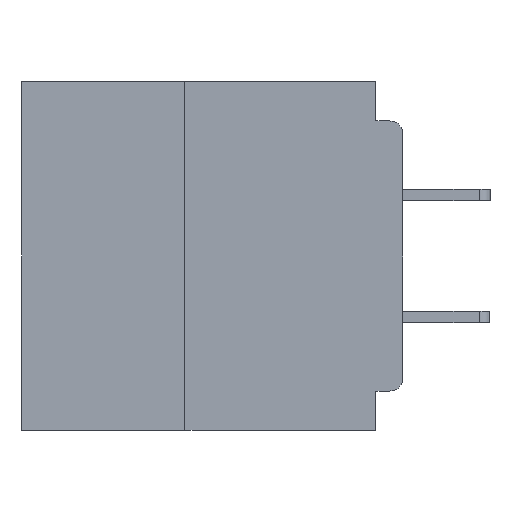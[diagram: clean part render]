
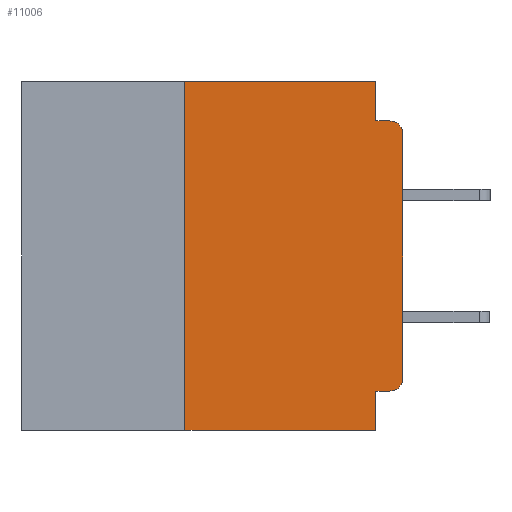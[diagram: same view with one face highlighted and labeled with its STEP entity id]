
A CAD part, left-side view. The second image highlights one B-rep face of the part: STEP entity #11006.
In plain terms, the highlighted planar face has unit normal (-1, 0, 0).
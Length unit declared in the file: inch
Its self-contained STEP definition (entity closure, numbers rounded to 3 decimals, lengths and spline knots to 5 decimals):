
#966 = CIRCLE ( 'NONE', #8583, 0.015 ) ;
#2147 = CARTESIAN_POINT ( 'NONE',  ( 0., 0.031, -0.045 ) ) ;
#2228 = ORIENTED_EDGE ( 'NONE', *, *, #18064, .T. ) ;
#3754 = CARTESIAN_POINT ( 'NONE',  ( 0., 0., -0.34 ) ) ;
#4077 = VERTEX_POINT ( 'NONE', #32138 ) ;
#4390 = LINE ( 'NONE', #18582, #49183 ) ;
#4826 = LINE ( 'NONE', #20694, #47069 ) ;
#5612 = CARTESIAN_POINT ( 'NONE',  ( 0., 0., -0.355 ) ) ;
#6241 = CARTESIAN_POINT ( 'NONE',  ( 0., 0.031, 0. ) ) ;
#7669 = ORIENTED_EDGE ( 'NONE', *, *, #29895, .F. ) ;
#7834 = LINE ( 'NONE', #51742, #28406 ) ;
#7839 = VERTEX_POINT ( 'NONE', #52609 ) ;
#7979 = LINE ( 'NONE', #29197, #25953 ) ;
#8038 = VECTOR ( 'NONE', #11817, 39.37008 ) ;
#8240 = EDGE_CURVE ( 'NONE', #22325, #8984, #49667, .T. ) ;
#8583 = AXIS2_PLACEMENT_3D ( 'NONE', #45046, #20536, #49139 ) ;
#8984 = VERTEX_POINT ( 'NONE', #2147 ) ;
#10341 = DIRECTION ( 'NONE',  ( 0., 0., -1. ) ) ;
#11006 = ADVANCED_FACE ( 'NONE', ( #14871 ), #15702, .F. ) ;
#11491 = AXIS2_PLACEMENT_3D ( 'NONE', #27928, #44354, #19817 ) ;
#11817 = DIRECTION ( 'NONE',  ( 0., -1., 0. ) ) ;
#12383 = LINE ( 'NONE', #46566, #24606 ) ;
#12419 = ORIENTED_EDGE ( 'NONE', *, *, #26550, .F. ) ;
#12953 = ORIENTED_EDGE ( 'NONE', *, *, #14827, .F. ) ;
#13663 = DIRECTION ( 'NONE',  ( 0., 1., 0. ) ) ;
#14096 = LINE ( 'NONE', #5612, #22427 ) ;
#14474 = CARTESIAN_POINT ( 'NONE',  ( 0., 0.015, -0.06 ) ) ;
#14827 = EDGE_CURVE ( 'NONE', #51454, #22325, #51598, .T. ) ;
#14871 = FACE_OUTER_BOUND ( 'NONE', #43298, .T. ) ;
#15254 = AXIS2_PLACEMENT_3D ( 'NONE', #14474, #43151, #18593 ) ;
#15267 = CARTESIAN_POINT ( 'NONE',  ( 0., 0.031, 0. ) ) ;
#15702 = PLANE ( 'NONE',  #11491 ) ;
#16562 = EDGE_CURVE ( 'NONE', #23070, #48485, #7834, .T. ) ;
#17034 = VECTOR ( 'NONE', #10341, 39.37008 ) ;
#18064 = EDGE_CURVE ( 'NONE', #48485, #38899, #24373, .T. ) ;
#18582 = CARTESIAN_POINT ( 'NONE',  ( 0., 0.031, -0.4 ) ) ;
#18593 = DIRECTION ( 'NONE',  ( 0., 0., -1. ) ) ;
#19001 = CARTESIAN_POINT ( 'NONE',  ( 0., 0.25, 0. ) ) ;
#19482 = ORIENTED_EDGE ( 'NONE', *, *, #27273, .F. ) ;
#19817 = DIRECTION ( 'NONE',  ( 0., 0., -1. ) ) ;
#20536 = DIRECTION ( 'NONE',  ( -1., 0., 0. ) ) ;
#20645 = CARTESIAN_POINT ( 'NONE',  ( 0., 0.031, -0.355 ) ) ;
#20694 = CARTESIAN_POINT ( 'NONE',  ( 0., 0., -0.045 ) ) ;
#20877 = DIRECTION ( 'NONE',  ( 0., -1., 0. ) ) ;
#22325 = VERTEX_POINT ( 'NONE', #15267 ) ;
#22427 = VECTOR ( 'NONE', #13663, 39.37008 ) ;
#22681 = DIRECTION ( 'NONE',  ( 0., 0., -1. ) ) ;
#23070 = VERTEX_POINT ( 'NONE', #3754 ) ;
#23648 = ORIENTED_EDGE ( 'NONE', *, *, #41224, .F. ) ;
#24373 = CIRCLE ( 'NONE', #15254, 0.015 ) ;
#24606 = VECTOR ( 'NONE', #26197, 39.37008 ) ;
#25038 = DIRECTION ( 'NONE',  ( 0., -1., 0. ) ) ;
#25953 = VECTOR ( 'NONE', #25038, 39.37008 ) ;
#26197 = DIRECTION ( 'NONE',  ( 0., 0., 1. ) ) ;
#26550 = EDGE_CURVE ( 'NONE', #8984, #38899, #4826, .T. ) ;
#27273 = EDGE_CURVE ( 'NONE', #4077, #51454, #12383, .T. ) ;
#27928 = CARTESIAN_POINT ( 'NONE',  ( 0., 0.437, 0. ) ) ;
#28406 = VECTOR ( 'NONE', #51565, 39.37008 ) ;
#29197 = CARTESIAN_POINT ( 'NONE',  ( 0., 0.437, -0.4 ) ) ;
#29895 = EDGE_CURVE ( 'NONE', #7839, #39234, #14096, .T. ) ;
#32138 = CARTESIAN_POINT ( 'NONE',  ( 0., 0.25, -0.4 ) ) ;
#38899 = VERTEX_POINT ( 'NONE', #43071 ) ;
#39124 = ORIENTED_EDGE ( 'NONE', *, *, #49460, .T. ) ;
#39234 = VERTEX_POINT ( 'NONE', #20645 ) ;
#41224 = EDGE_CURVE ( 'NONE', #39234, #43270, #4390, .T. ) ;
#43071 = CARTESIAN_POINT ( 'NONE',  ( 0., 0.015, -0.045 ) ) ;
#43151 = DIRECTION ( 'NONE',  ( -1., 0., 0. ) ) ;
#43270 = VERTEX_POINT ( 'NONE', #52366 ) ;
#43298 = EDGE_LOOP ( 'NONE', ( #47758, #2228, #12419, #45518, #12953, #19482, #45007, #23648, #7669, #39124 ) ) ;
#44354 = DIRECTION ( 'NONE',  ( 1., 0., 0. ) ) ;
#45007 = ORIENTED_EDGE ( 'NONE', *, *, #52684, .T. ) ;
#45046 = CARTESIAN_POINT ( 'NONE',  ( 0., 0.015, -0.34 ) ) ;
#45518 = ORIENTED_EDGE ( 'NONE', *, *, #8240, .F. ) ;
#46566 = CARTESIAN_POINT ( 'NONE',  ( 0., 0.25, -0.4 ) ) ;
#47069 = VECTOR ( 'NONE', #20877, 39.37008 ) ;
#47758 = ORIENTED_EDGE ( 'NONE', *, *, #16562, .T. ) ;
#48485 = VERTEX_POINT ( 'NONE', #50851 ) ;
#48703 = CARTESIAN_POINT ( 'NONE',  ( 0., 0.437, 0. ) ) ;
#49139 = DIRECTION ( 'NONE',  ( 0., 0., -1. ) ) ;
#49183 = VECTOR ( 'NONE', #22681, 39.37008 ) ;
#49460 = EDGE_CURVE ( 'NONE', #7839, #23070, #966, .T. ) ;
#49667 = LINE ( 'NONE', #6241, #17034 ) ;
#50851 = CARTESIAN_POINT ( 'NONE',  ( 0., 0., -0.06 ) ) ;
#51454 = VERTEX_POINT ( 'NONE', #19001 ) ;
#51565 = DIRECTION ( 'NONE',  ( 0., 0., 1. ) ) ;
#51598 = LINE ( 'NONE', #48703, #8038 ) ;
#51742 = CARTESIAN_POINT ( 'NONE',  ( 0., 0., 0. ) ) ;
#52366 = CARTESIAN_POINT ( 'NONE',  ( 0., 0.031, -0.4 ) ) ;
#52609 = CARTESIAN_POINT ( 'NONE',  ( 0., 0.015, -0.355 ) ) ;
#52684 = EDGE_CURVE ( 'NONE', #4077, #43270, #7979, .T. ) ;
